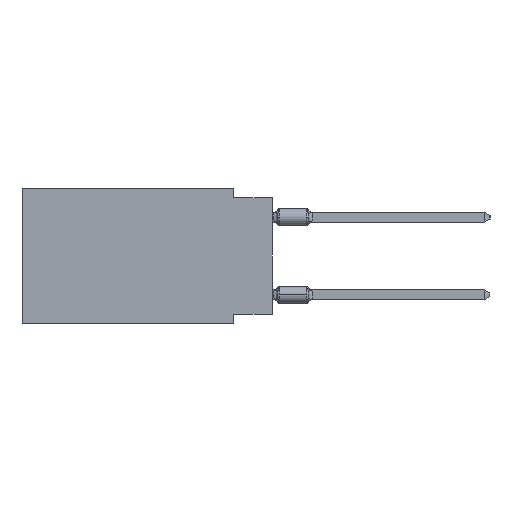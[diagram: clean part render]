
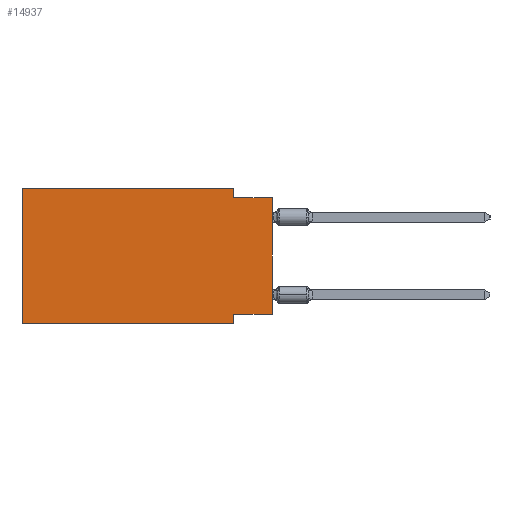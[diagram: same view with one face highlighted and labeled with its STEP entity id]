
A CAD part, left-side view. The second image highlights one B-rep face of the part: STEP entity #14937.
In plain terms, the highlighted planar face has unit normal (-1, 0, 0).
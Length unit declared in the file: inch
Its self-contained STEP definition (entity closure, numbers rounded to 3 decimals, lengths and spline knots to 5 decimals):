
#240 = LINE ( 'NONE', #32515, #9596 ) ;
#734 = VECTOR ( 'NONE', #1929, 39.37008 ) ;
#1032 = CARTESIAN_POINT ( 'NONE',  ( 0., 0.645, 0. ) ) ;
#1713 = VECTOR ( 'NONE', #17549, 39.37008 ) ;
#1929 = DIRECTION ( 'NONE',  ( 0., 0., 1. ) ) ;
#3616 = PLANE ( 'NONE',  #23927 ) ;
#3794 = DIRECTION ( 'NONE',  ( 1., 0., 0. ) ) ;
#4035 = VERTEX_POINT ( 'NONE', #9845 ) ;
#4196 = LINE ( 'NONE', #24237, #734 ) ;
#4198 = DIRECTION ( 'NONE',  ( 0., 0., -1. ) ) ;
#4421 = LINE ( 'NONE', #1032, #29998 ) ;
#5015 = EDGE_CURVE ( 'NONE', #12945, #4035, #240, .T. ) ;
#5756 = LINE ( 'NONE', #17645, #28668 ) ;
#6331 = EDGE_CURVE ( 'NONE', #36944, #32412, #35112, .T. ) ;
#6871 = ORIENTED_EDGE ( 'NONE', *, *, #32948, .F. ) ;
#8428 = CARTESIAN_POINT ( 'NONE',  ( 0., 0.645, 0. ) ) ;
#9359 = CARTESIAN_POINT ( 'NONE',  ( 0., 0.645, -0.35 ) ) ;
#9596 = VECTOR ( 'NONE', #17626, 39.37008 ) ;
#9845 = CARTESIAN_POINT ( 'NONE',  ( 0., 0.1, -0.325 ) ) ;
#10372 = EDGE_CURVE ( 'NONE', #12945, #24390, #4196, .T. ) ;
#10488 = VECTOR ( 'NONE', #12388, 39.37008 ) ;
#11234 = ORIENTED_EDGE ( 'NONE', *, *, #31324, .T. ) ;
#12388 = DIRECTION ( 'NONE',  ( 0., -1., 0. ) ) ;
#12945 = VERTEX_POINT ( 'NONE', #31999 ) ;
#14561 = CARTESIAN_POINT ( 'NONE',  ( 0., 0.1, 0. ) ) ;
#14937 = ADVANCED_FACE ( 'NONE', ( #18539 ), #3616, .F. ) ;
#14962 = CARTESIAN_POINT ( 'NONE',  ( 0., 0.645, 0. ) ) ;
#15962 = DIRECTION ( 'NONE',  ( 0., -1., 0. ) ) ;
#17549 = DIRECTION ( 'NONE',  ( 0., 0., 1. ) ) ;
#17626 = DIRECTION ( 'NONE',  ( 0., 1., 0. ) ) ;
#17645 = CARTESIAN_POINT ( 'NONE',  ( 0., 0.1, -0.35 ) ) ;
#17833 = VERTEX_POINT ( 'NONE', #8428 ) ;
#18052 = EDGE_CURVE ( 'NONE', #17833, #36944, #4421, .T. ) ;
#18352 = DIRECTION ( 'NONE',  ( 0., 0., -1. ) ) ;
#18539 = FACE_OUTER_BOUND ( 'NONE', #22763, .T. ) ;
#18621 = LINE ( 'NONE', #9359, #10488 ) ;
#19088 = LINE ( 'NONE', #19276, #23880 ) ;
#19276 = CARTESIAN_POINT ( 'NONE',  ( 0., 0., -0.025 ) ) ;
#19439 = ORIENTED_EDGE ( 'NONE', *, *, #6331, .F. ) ;
#19857 = ORIENTED_EDGE ( 'NONE', *, *, #10372, .T. ) ;
#20746 = ORIENTED_EDGE ( 'NONE', *, *, #30512, .F. ) ;
#20783 = DIRECTION ( 'NONE',  ( 0., 0., -1. ) ) ;
#21207 = CARTESIAN_POINT ( 'NONE',  ( 0., 0.645, -0.35 ) ) ;
#21876 = ORIENTED_EDGE ( 'NONE', *, *, #5015, .F. ) ;
#21927 = DIRECTION ( 'NONE',  ( 0., -1., 0. ) ) ;
#22763 = EDGE_LOOP ( 'NONE', ( #19857, #20746, #19439, #34549, #26773, #11234, #6871, #21876 ) ) ;
#23083 = VECTOR ( 'NONE', #20783, 39.37008 ) ;
#23336 = VERTEX_POINT ( 'NONE', #24777 ) ;
#23880 = VECTOR ( 'NONE', #21927, 39.37008 ) ;
#23927 = AXIS2_PLACEMENT_3D ( 'NONE', #14962, #3794, #18352 ) ;
#24237 = CARTESIAN_POINT ( 'NONE',  ( 0., 0., 0. ) ) ;
#24390 = VERTEX_POINT ( 'NONE', #26132 ) ;
#24777 = CARTESIAN_POINT ( 'NONE',  ( 0., 0.1, -0.35 ) ) ;
#26132 = CARTESIAN_POINT ( 'NONE',  ( 0., 0., -0.025 ) ) ;
#26188 = CARTESIAN_POINT ( 'NONE',  ( 0., 0.1, -0.025 ) ) ;
#26707 = EDGE_CURVE ( 'NONE', #36920, #17833, #31525, .T. ) ;
#26773 = ORIENTED_EDGE ( 'NONE', *, *, #26707, .F. ) ;
#28668 = VECTOR ( 'NONE', #4198, 39.37008 ) ;
#28895 = CARTESIAN_POINT ( 'NONE',  ( 0., 0.645, 0. ) ) ;
#29507 = CARTESIAN_POINT ( 'NONE',  ( 0., 0.1, 0. ) ) ;
#29998 = VECTOR ( 'NONE', #15962, 39.37008 ) ;
#30512 = EDGE_CURVE ( 'NONE', #32412, #24390, #19088, .T. ) ;
#31324 = EDGE_CURVE ( 'NONE', #36920, #23336, #18621, .T. ) ;
#31525 = LINE ( 'NONE', #28895, #1713 ) ;
#31999 = CARTESIAN_POINT ( 'NONE',  ( 0., 0., -0.325 ) ) ;
#32412 = VERTEX_POINT ( 'NONE', #26188 ) ;
#32515 = CARTESIAN_POINT ( 'NONE',  ( 0., 0., -0.325 ) ) ;
#32948 = EDGE_CURVE ( 'NONE', #4035, #23336, #5756, .T. ) ;
#34549 = ORIENTED_EDGE ( 'NONE', *, *, #18052, .F. ) ;
#35112 = LINE ( 'NONE', #14561, #23083 ) ;
#36920 = VERTEX_POINT ( 'NONE', #21207 ) ;
#36944 = VERTEX_POINT ( 'NONE', #29507 ) ;
